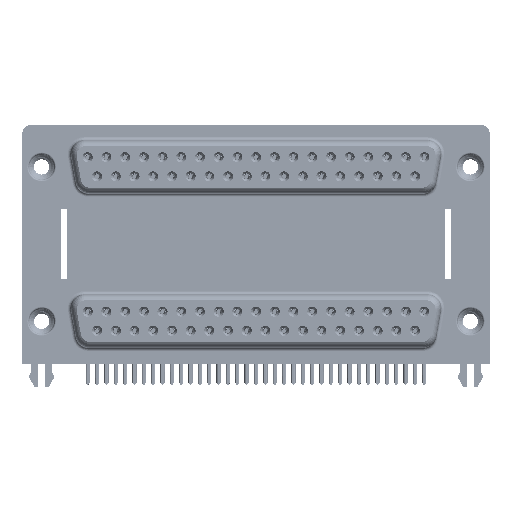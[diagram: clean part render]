
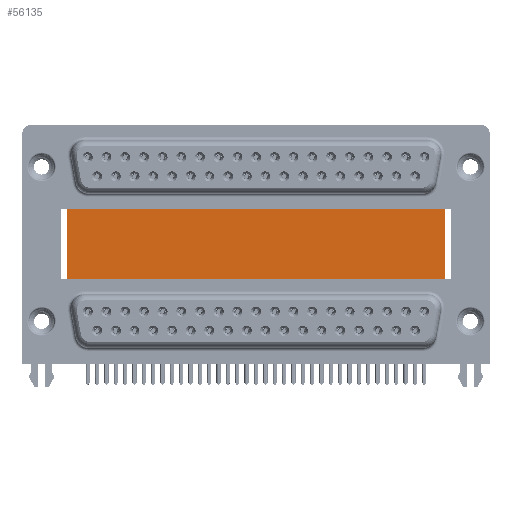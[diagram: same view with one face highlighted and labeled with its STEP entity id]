
A CAD part, top view. The second image highlights one B-rep face of the part: STEP entity #56135.
In plain terms, the highlighted planar face has unit normal (0, 0, 1).
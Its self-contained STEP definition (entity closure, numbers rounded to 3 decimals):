
#1332 = DIRECTION ( 'NONE',  ( -1., 0., 0. ) ) ;
#2506 = CARTESIAN_POINT ( 'NONE',  ( 59.71, 16.585, -12. ) ) ;
#2891 = CARTESIAN_POINT ( 'NONE',  ( 3.79, 16.585, -12. ) ) ;
#4467 = VECTOR ( 'NONE', #63961, 1000. ) ;
#7945 = FACE_OUTER_BOUND ( 'NONE', #31885, .T. ) ;
#13079 = ORIENTED_EDGE ( 'NONE', *, *, #51285, .F. ) ;
#13182 = VERTEX_POINT ( 'NONE', #2506 ) ;
#14332 = VERTEX_POINT ( 'NONE', #46535 ) ;
#17278 = DIRECTION ( 'NONE',  ( 0., -1., 0. ) ) ;
#19648 = PLANE ( 'NONE',  #42343 ) ;
#26040 = VECTOR ( 'NONE', #28686, 1000. ) ;
#28111 = LINE ( 'NONE', #70184, #4467 ) ;
#28686 = DIRECTION ( 'NONE',  ( 1., 0., 0. ) ) ;
#31579 = EDGE_CURVE ( 'NONE', #57974, #13182, #38400, .T. ) ;
#31885 = EDGE_LOOP ( 'NONE', ( #72823, #13079, #67127, #67260 ) ) ;
#35685 = CARTESIAN_POINT ( 'NONE',  ( 3.79, -3.735, -12. ) ) ;
#37599 = DIRECTION ( 'NONE',  ( 0., 0., -1. ) ) ;
#38400 = LINE ( 'NONE', #2891, #50728 ) ;
#42343 = AXIS2_PLACEMENT_3D ( 'NONE', #66070, #37599, #1332 ) ;
#46155 = LINE ( 'NONE', #71422, #49407 ) ;
#46535 = CARTESIAN_POINT ( 'NONE',  ( 3.79, -3.735, -12. ) ) ;
#46989 = LINE ( 'NONE', #35685, #26040 ) ;
#49216 = CARTESIAN_POINT ( 'NONE',  ( 3.79, 16.585, -12. ) ) ;
#49407 = VECTOR ( 'NONE', #17278, 1000. ) ;
#50728 = VECTOR ( 'NONE', #56690, 1000. ) ;
#50842 = EDGE_CURVE ( 'NONE', #57974, #14332, #46155, .T. ) ;
#51285 = EDGE_CURVE ( 'NONE', #13182, #55484, #28111, .T. ) ;
#55484 = VERTEX_POINT ( 'NONE', #73699 ) ;
#56135 = ADVANCED_FACE ( 'NONE', ( #7945 ), #19648, .F. ) ;
#56690 = DIRECTION ( 'NONE',  ( 1., 0., 0. ) ) ;
#57974 = VERTEX_POINT ( 'NONE', #49216 ) ;
#63961 = DIRECTION ( 'NONE',  ( 0., -1., 0. ) ) ;
#66070 = CARTESIAN_POINT ( 'NONE',  ( 3.79, 16.585, -12. ) ) ;
#67127 = ORIENTED_EDGE ( 'NONE', *, *, #31579, .F. ) ;
#67260 = ORIENTED_EDGE ( 'NONE', *, *, #50842, .T. ) ;
#67349 = EDGE_CURVE ( 'NONE', #14332, #55484, #46989, .T. ) ;
#70184 = CARTESIAN_POINT ( 'NONE',  ( 59.71, 16.585, -12. ) ) ;
#71422 = CARTESIAN_POINT ( 'NONE',  ( 3.79, 16.585, -12. ) ) ;
#72823 = ORIENTED_EDGE ( 'NONE', *, *, #67349, .T. ) ;
#73699 = CARTESIAN_POINT ( 'NONE',  ( 59.71, -3.735, -12. ) ) ;
